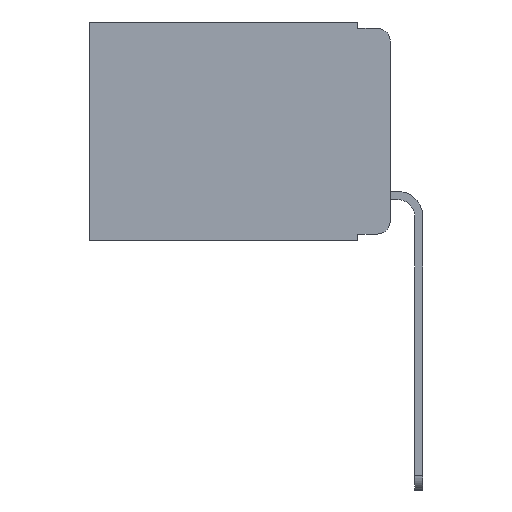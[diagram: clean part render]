
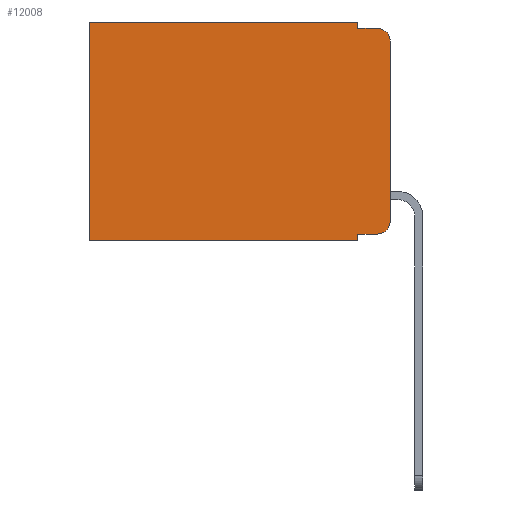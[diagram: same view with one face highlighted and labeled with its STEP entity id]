
A CAD part, left-side view. The second image highlights one B-rep face of the part: STEP entity #12008.
In plain terms, the highlighted planar face has unit normal (-1, 0, 0).
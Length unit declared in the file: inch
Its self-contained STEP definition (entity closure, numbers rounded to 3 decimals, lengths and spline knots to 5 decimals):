
#111 = ORIENTED_EDGE ( 'NONE', *, *, #445, .T. ) ;
#426 = DIRECTION ( 'NONE',  ( 0., -1., 0. ) ) ;
#445 = EDGE_CURVE ( 'NONE', #7935, #13762, #13721, .T. ) ;
#1070 = CARTESIAN_POINT ( 'NONE',  ( 0.298, 0.051, 0. ) ) ;
#1307 = CARTESIAN_POINT ( 'NONE',  ( 0.298, 0.473, -0.343 ) ) ;
#1339 = VECTOR ( 'NONE', #426, 39.37008 ) ;
#1832 = CARTESIAN_POINT ( 'NONE',  ( 0.298, 0.02, -0.01 ) ) ;
#2174 = DIRECTION ( 'NONE',  ( 0., 1., 0. ) ) ;
#2283 = VECTOR ( 'NONE', #5350, 39.37008 ) ;
#2595 = VECTOR ( 'NONE', #2610, 39.37008 ) ;
#2610 = DIRECTION ( 'NONE',  ( 0., 0., -1. ) ) ;
#2655 = CARTESIAN_POINT ( 'NONE',  ( 0.298, 0.02, -0.333 ) ) ;
#3009 = EDGE_CURVE ( 'NONE', #5417, #10143, #8054, .T. ) ;
#4085 = VECTOR ( 'NONE', #2174, 39.37008 ) ;
#4125 = EDGE_CURVE ( 'NONE', #11354, #4653, #5222, .T. ) ;
#4206 = ORIENTED_EDGE ( 'NONE', *, *, #3009, .F. ) ;
#4214 = CARTESIAN_POINT ( 'NONE',  ( 0.298, 0., 0. ) ) ;
#4250 = DIRECTION ( 'NONE',  ( 0., -1., 0. ) ) ;
#4298 = ORIENTED_EDGE ( 'NONE', *, *, #9126, .T. ) ;
#4392 = AXIS2_PLACEMENT_3D ( 'NONE', #9583, #12021, #6649 ) ;
#4653 = VERTEX_POINT ( 'NONE', #2655 ) ;
#4906 = VERTEX_POINT ( 'NONE', #8732 ) ;
#4920 = LINE ( 'NONE', #9957, #2595 ) ;
#4988 = ORIENTED_EDGE ( 'NONE', *, *, #7382, .F. ) ;
#5042 = VECTOR ( 'NONE', #13412, 39.37008 ) ;
#5047 = VECTOR ( 'NONE', #10588, 39.37008 ) ;
#5222 = LINE ( 'NONE', #5495, #12708 ) ;
#5350 = DIRECTION ( 'NONE',  ( 0., 0., -1. ) ) ;
#5417 = VERTEX_POINT ( 'NONE', #8647 ) ;
#5495 = CARTESIAN_POINT ( 'NONE',  ( 0.298, 0.051, -0.333 ) ) ;
#5565 = CARTESIAN_POINT ( 'NONE',  ( 0.298, 0., 0. ) ) ;
#5661 = CARTESIAN_POINT ( 'NONE',  ( 0.298, 0.051, 0. ) ) ;
#5851 = EDGE_CURVE ( 'NONE', #7935, #5417, #6402, .T. ) ;
#6289 = DIRECTION ( 'NONE',  ( -1., 0., 0. ) ) ;
#6402 = LINE ( 'NONE', #1070, #2283 ) ;
#6649 = DIRECTION ( 'NONE',  ( 0., 0., -1. ) ) ;
#6712 = LINE ( 'NONE', #5661, #5042 ) ;
#6949 = CARTESIAN_POINT ( 'NONE',  ( 0.298, 0.051, -0.333 ) ) ;
#7268 = CARTESIAN_POINT ( 'NONE',  ( 0.298, 0.02, -0.313 ) ) ;
#7382 = EDGE_CURVE ( 'NONE', #11855, #4906, #11013, .T. ) ;
#7485 = AXIS2_PLACEMENT_3D ( 'NONE', #7268, #6289, #13831 ) ;
#7926 = CARTESIAN_POINT ( 'NONE',  ( 0.298, 0.051, -0.01 ) ) ;
#7935 = VERTEX_POINT ( 'NONE', #13421 ) ;
#7994 = EDGE_CURVE ( 'NONE', #4653, #4906, #8821, .T. ) ;
#8053 = VERTEX_POINT ( 'NONE', #1307 ) ;
#8054 = LINE ( 'NONE', #7926, #1339 ) ;
#8341 = CARTESIAN_POINT ( 'NONE',  ( 0.298, 0.02, -0.03 ) ) ;
#8548 = DIRECTION ( 'NONE',  ( 0., 0., -1. ) ) ;
#8647 = CARTESIAN_POINT ( 'NONE',  ( 0.298, 0.051, -0.01 ) ) ;
#8732 = CARTESIAN_POINT ( 'NONE',  ( 0.298, 0., -0.313 ) ) ;
#8755 = EDGE_CURVE ( 'NONE', #9886, #8053, #11089, .T. ) ;
#8821 = CIRCLE ( 'NONE', #7485, 0.02 ) ;
#9126 = EDGE_CURVE ( 'NONE', #13762, #8053, #4920, .T. ) ;
#9526 = ORIENTED_EDGE ( 'NONE', *, *, #7994, .T. ) ;
#9583 = CARTESIAN_POINT ( 'NONE',  ( 0.298, 0., 0. ) ) ;
#9886 = VERTEX_POINT ( 'NONE', #11559 ) ;
#9957 = CARTESIAN_POINT ( 'NONE',  ( 0.298, 0.473, 0. ) ) ;
#10143 = VERTEX_POINT ( 'NONE', #1832 ) ;
#10161 = ORIENTED_EDGE ( 'NONE', *, *, #11565, .T. ) ;
#10178 = EDGE_LOOP ( 'NONE', ( #4988, #10161, #4206, #12770, #111, #4298, #10389, #10229, #12203, #9526 ) ) ;
#10183 = AXIS2_PLACEMENT_3D ( 'NONE', #8341, #13805, #8548 ) ;
#10229 = ORIENTED_EDGE ( 'NONE', *, *, #10985, .F. ) ;
#10389 = ORIENTED_EDGE ( 'NONE', *, *, #8755, .F. ) ;
#10588 = DIRECTION ( 'NONE',  ( 0., 1., 0. ) ) ;
#10907 = FACE_OUTER_BOUND ( 'NONE', #10178, .T. ) ;
#10985 = EDGE_CURVE ( 'NONE', #11354, #9886, #6712, .T. ) ;
#11013 = LINE ( 'NONE', #5565, #13057 ) ;
#11089 = LINE ( 'NONE', #13813, #5047 ) ;
#11354 = VERTEX_POINT ( 'NONE', #6949 ) ;
#11559 = CARTESIAN_POINT ( 'NONE',  ( 0.298, 0.051, -0.343 ) ) ;
#11565 = EDGE_CURVE ( 'NONE', #11855, #10143, #12189, .T. ) ;
#11855 = VERTEX_POINT ( 'NONE', #13573 ) ;
#12008 = ADVANCED_FACE ( 'NONE', ( #10907 ), #12873, .F. ) ;
#12021 = DIRECTION ( 'NONE',  ( 1., 0., 0. ) ) ;
#12189 = CIRCLE ( 'NONE', #10183, 0.02 ) ;
#12203 = ORIENTED_EDGE ( 'NONE', *, *, #4125, .T. ) ;
#12708 = VECTOR ( 'NONE', #4250, 39.37008 ) ;
#12770 = ORIENTED_EDGE ( 'NONE', *, *, #5851, .F. ) ;
#12779 = CARTESIAN_POINT ( 'NONE',  ( 0.298, 0.473, 0. ) ) ;
#12873 = PLANE ( 'NONE',  #4392 ) ;
#13052 = DIRECTION ( 'NONE',  ( 0., 0., -1. ) ) ;
#13057 = VECTOR ( 'NONE', #13052, 39.37008 ) ;
#13412 = DIRECTION ( 'NONE',  ( 0., 0., -1. ) ) ;
#13421 = CARTESIAN_POINT ( 'NONE',  ( 0.298, 0.051, 0. ) ) ;
#13573 = CARTESIAN_POINT ( 'NONE',  ( 0.298, 0., -0.03 ) ) ;
#13721 = LINE ( 'NONE', #4214, #4085 ) ;
#13762 = VERTEX_POINT ( 'NONE', #12779 ) ;
#13805 = DIRECTION ( 'NONE',  ( -1., 0., 0. ) ) ;
#13813 = CARTESIAN_POINT ( 'NONE',  ( 0.298, 0., -0.343 ) ) ;
#13831 = DIRECTION ( 'NONE',  ( 0., 0., -1. ) ) ;
